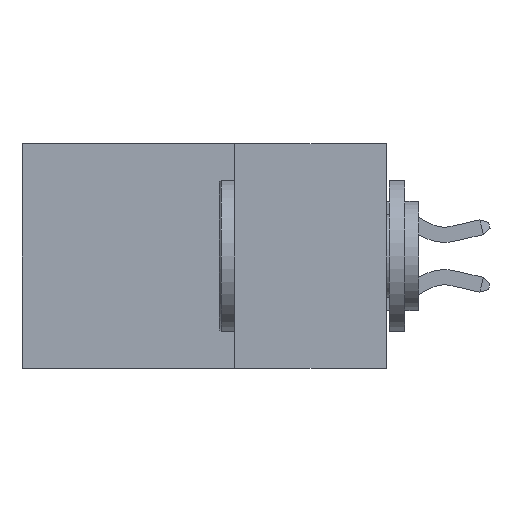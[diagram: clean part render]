
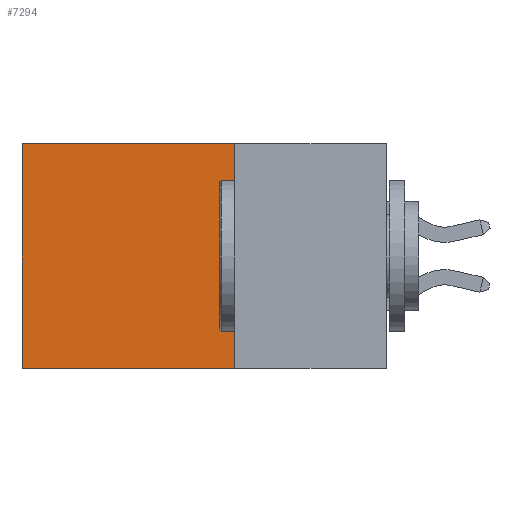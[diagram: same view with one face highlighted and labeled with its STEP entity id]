
A CAD part, left-side view. The second image highlights one B-rep face of the part: STEP entity #7294.
In plain terms, the highlighted planar face has unit normal (-1, 0, 0).
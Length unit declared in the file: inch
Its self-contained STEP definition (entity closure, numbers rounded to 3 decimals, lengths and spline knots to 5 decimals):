
#437 = CARTESIAN_POINT ( 'NONE',  ( 0.2615, 0.25, -0.37 ) ) ;
#1160 = VERTEX_POINT ( 'NONE', #6476 ) ;
#1308 = VERTEX_POINT ( 'NONE', #10884 ) ;
#1419 = ORIENTED_EDGE ( 'NONE', *, *, #6736, .T. ) ;
#1659 = DIRECTION ( 'NONE',  ( 0., 1., 0. ) ) ;
#2136 = LINE ( 'NONE', #9531, #4029 ) ;
#2557 = DIRECTION ( 'NONE',  ( 0., 1., 0. ) ) ;
#2577 = LINE ( 'NONE', #8163, #11258 ) ;
#3100 = DIRECTION ( 'NONE',  ( 1., 0., 0. ) ) ;
#3540 = CARTESIAN_POINT ( 'NONE',  ( 0.2615, 0.25, 0. ) ) ;
#3887 = ORIENTED_EDGE ( 'NONE', *, *, #7451, .T. ) ;
#4029 = VECTOR ( 'NONE', #9418, 39.37008 ) ;
#4638 = ORIENTED_EDGE ( 'NONE', *, *, #11448, .F. ) ;
#5032 = PLANE ( 'NONE',  #11024 ) ;
#5504 = EDGE_CURVE ( 'NONE', #7484, #1160, #2136, .T. ) ;
#6181 = VECTOR ( 'NONE', #2557, 39.37008 ) ;
#6183 = LINE ( 'NONE', #3540, #6181 ) ;
#6430 = CARTESIAN_POINT ( 'NONE',  ( 0.2615, 0.6, 0. ) ) ;
#6476 = CARTESIAN_POINT ( 'NONE',  ( 0.2615, 0.25, -0.37 ) ) ;
#6736 = EDGE_CURVE ( 'NONE', #11890, #1308, #11797, .T. ) ;
#7161 = EDGE_LOOP ( 'NONE', ( #1419, #4638, #8508, #3887 ) ) ;
#7197 = CARTESIAN_POINT ( 'NONE',  ( 0.2615, 0.6, -0.37 ) ) ;
#7286 = CARTESIAN_POINT ( 'NONE',  ( 0.2615, 0.25, 0. ) ) ;
#7294 = ADVANCED_FACE ( 'NONE', ( #10481 ), #5032, .F. ) ;
#7451 = EDGE_CURVE ( 'NONE', #7484, #11890, #6183, .T. ) ;
#7484 = VERTEX_POINT ( 'NONE', #7286 ) ;
#8163 = CARTESIAN_POINT ( 'NONE',  ( 0.2615, 0.25, -0.37 ) ) ;
#8508 = ORIENTED_EDGE ( 'NONE', *, *, #5504, .F. ) ;
#9418 = DIRECTION ( 'NONE',  ( 0., 0., -1. ) ) ;
#9460 = VECTOR ( 'NONE', #10881, 39.37008 ) ;
#9531 = CARTESIAN_POINT ( 'NONE',  ( 0.2615, 0.25, -0.37 ) ) ;
#9696 = DIRECTION ( 'NONE',  ( 0., 0., -1. ) ) ;
#10481 = FACE_OUTER_BOUND ( 'NONE', #7161, .T. ) ;
#10881 = DIRECTION ( 'NONE',  ( 0., 0., -1. ) ) ;
#10884 = CARTESIAN_POINT ( 'NONE',  ( 0.2615, 0.6, -0.37 ) ) ;
#11024 = AXIS2_PLACEMENT_3D ( 'NONE', #437, #3100, #9696 ) ;
#11258 = VECTOR ( 'NONE', #1659, 39.37008 ) ;
#11448 = EDGE_CURVE ( 'NONE', #1160, #1308, #2577, .T. ) ;
#11797 = LINE ( 'NONE', #7197, #9460 ) ;
#11890 = VERTEX_POINT ( 'NONE', #6430 ) ;
